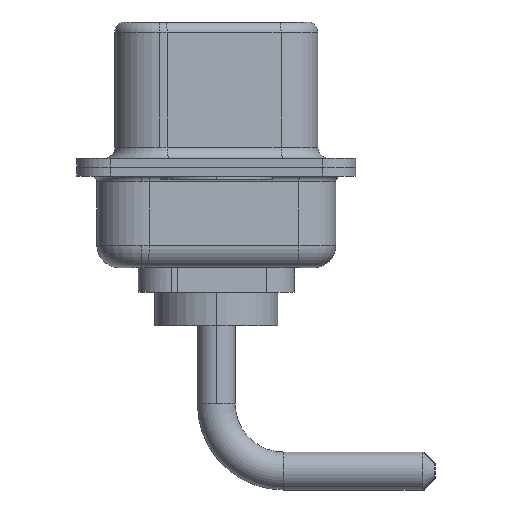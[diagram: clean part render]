
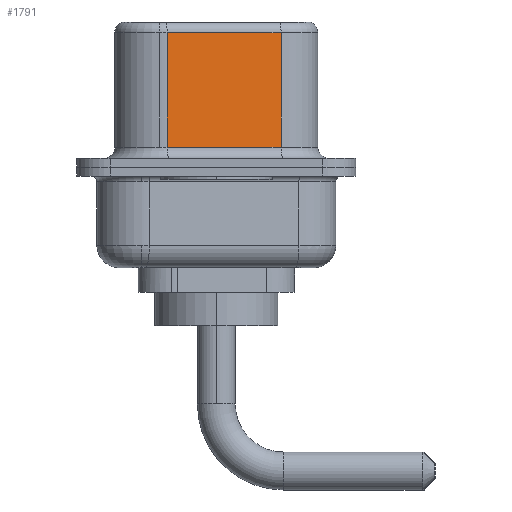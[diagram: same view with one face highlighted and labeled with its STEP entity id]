
A CAD part, left-side view. The second image highlights one B-rep face of the part: STEP entity #1791.
In plain terms, the highlighted planar face has unit normal (-0.985, -0.174, 0).
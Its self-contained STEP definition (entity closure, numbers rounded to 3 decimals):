
#941 = LINE ( 'NONE', #9641, #3740 ) ;
#1791 = ADVANCED_FACE ( 'NONE', ( #9120 ), #4289, .F. ) ;
#1914 = VERTEX_POINT ( 'NONE', #6085 ) ;
#2291 = EDGE_CURVE ( 'NONE', #11765, #8959, #3865, .T. ) ;
#2330 = VECTOR ( 'NONE', #6115, 1000. ) ;
#3131 = CARTESIAN_POINT ( 'NONE',  ( 3.68, 2.203, 6.52 ) ) ;
#3328 = ORIENTED_EDGE ( 'NONE', *, *, #5056, .T. ) ;
#3342 = CARTESIAN_POINT ( 'NONE',  ( 4.58, -2.897, 6.52 ) ) ;
#3740 = VECTOR ( 'NONE', #11546, 1000. ) ;
#3784 = CARTESIAN_POINT ( 'NONE',  ( 4.58, -2.897, 6.02 ) ) ;
#3865 = LINE ( 'NONE', #7866, #10758 ) ;
#4289 = PLANE ( 'NONE',  #9738 ) ;
#5056 = EDGE_CURVE ( 'NONE', #12124, #1914, #10101, .T. ) ;
#5184 = CARTESIAN_POINT ( 'NONE',  ( 4.58, -2.897, 6.02 ) ) ;
#5241 = LINE ( 'NONE', #5184, #9565 ) ;
#5263 = ORIENTED_EDGE ( 'NONE', *, *, #9441, .T. ) ;
#6085 = CARTESIAN_POINT ( 'NONE',  ( 3.68, 2.203, 0.9 ) ) ;
#6115 = DIRECTION ( 'NONE',  ( 0., 0., -1. ) ) ;
#6275 = CARTESIAN_POINT ( 'NONE',  ( 4.58, -2.897, 0.9 ) ) ;
#6376 = ORIENTED_EDGE ( 'NONE', *, *, #2291, .F. ) ;
#6502 = CARTESIAN_POINT ( 'NONE',  ( 3.68, 2.203, 6.02 ) ) ;
#6513 = DIRECTION ( 'NONE',  ( 0.985, 0.174, 0. ) ) ;
#7866 = CARTESIAN_POINT ( 'NONE',  ( 4.58, -2.897, 6.52 ) ) ;
#8286 = DIRECTION ( 'NONE',  ( -0.174, 0.985, 0. ) ) ;
#8959 = VERTEX_POINT ( 'NONE', #6275 ) ;
#9120 = FACE_OUTER_BOUND ( 'NONE', #12439, .T. ) ;
#9421 = DIRECTION ( 'NONE',  ( -0.174, 0.985, 0. ) ) ;
#9441 = EDGE_CURVE ( 'NONE', #11765, #12124, #5241, .T. ) ;
#9565 = VECTOR ( 'NONE', #8286, 1000. ) ;
#9641 = CARTESIAN_POINT ( 'NONE',  ( 4.58, -2.897, 0.9 ) ) ;
#9669 = ORIENTED_EDGE ( 'NONE', *, *, #11429, .T. ) ;
#9738 = AXIS2_PLACEMENT_3D ( 'NONE', #3342, #6513, #9421 ) ;
#10101 = LINE ( 'NONE', #3131, #2330 ) ;
#10758 = VECTOR ( 'NONE', #11720, 1000. ) ;
#11429 = EDGE_CURVE ( 'NONE', #1914, #8959, #941, .T. ) ;
#11546 = DIRECTION ( 'NONE',  ( 0.174, -0.985, 0. ) ) ;
#11720 = DIRECTION ( 'NONE',  ( 0., 0., -1. ) ) ;
#11765 = VERTEX_POINT ( 'NONE', #3784 ) ;
#12124 = VERTEX_POINT ( 'NONE', #6502 ) ;
#12439 = EDGE_LOOP ( 'NONE', ( #6376, #5263, #3328, #9669 ) ) ;
